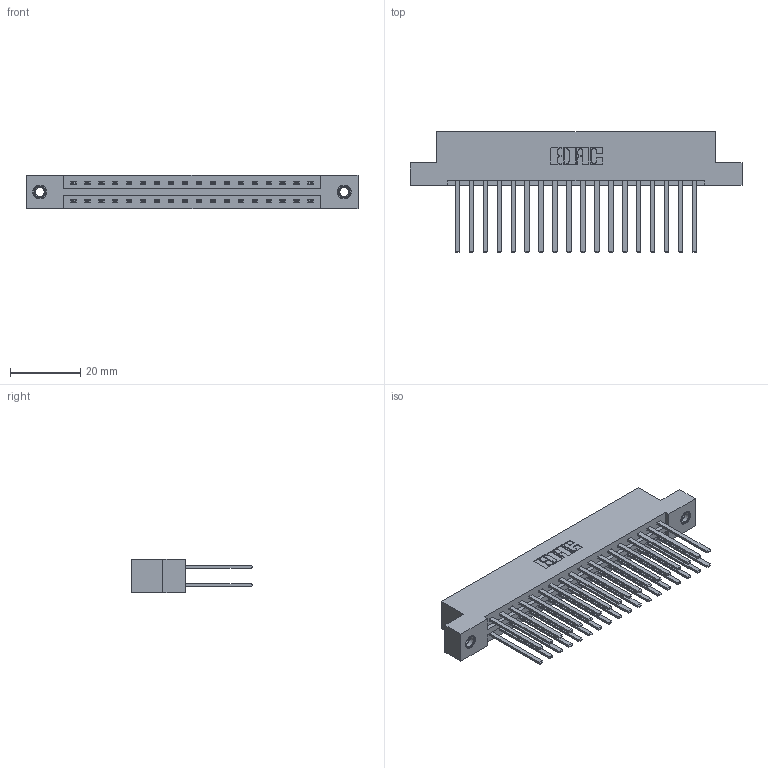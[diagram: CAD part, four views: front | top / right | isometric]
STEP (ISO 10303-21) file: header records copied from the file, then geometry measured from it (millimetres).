
FILE_DESCRIPTION (( 'STEP AP203' ), '1' );
FILE_NAME ('337-036-544-207.STEP', '2019-10-08T21:00:55', ( '' ), ( '' ), 'SwSTEP 2.0', 'SolidWorks 2016', '' );
FILE_SCHEMA (( 'CONFIG_CONTROL_DESIGN' ));
Length unit declared in the file: inch
Products named in the file (4): 345-292-001_345-293-144; 337-036-544-207; 337 Part_Flush Mounting Lugs - 0.156 Dia-TI; 345-250-001_345-250-005-103
Assembly tree (39 placements, depth 2):
  337-036-544-207
    337 Part_Flush Mounting Lugs - 0.156 Dia-TI
    345-292-001_345-293-144  x36
    345-250-001_345-250-005-103  x2
Bounding box: 94.34 x 34.3 x 9.4 mm (x, y, z)
Volume: 10113.5 mm3; surface area: 12884.7 mm2
Topology: 39 solids, 39 shells, 1902 faces, 5595 edges, 3674 vertices
Faces by surface type: plane 1326, cylinder 560, cone 12, torus 4
Entity records: 18062 total; most frequent: CARTESIAN_POINT 3041, ORIENTED_EDGE 2970, DIRECTION 2659, EDGE_CURVE 1485, VECTOR 1341, LINE 1341, VERTEX_POINT 984, AXIS2_PLACEMENT_3D 659
